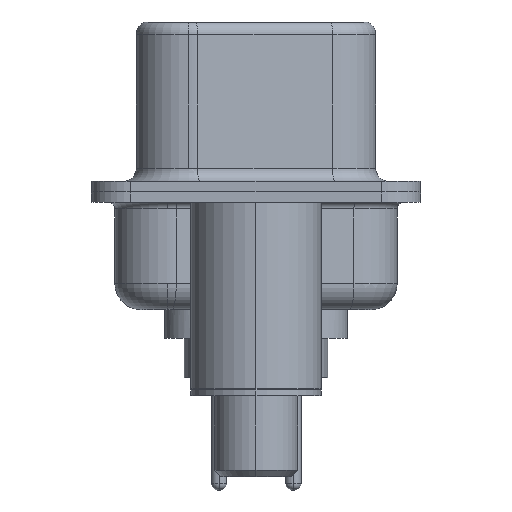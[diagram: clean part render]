
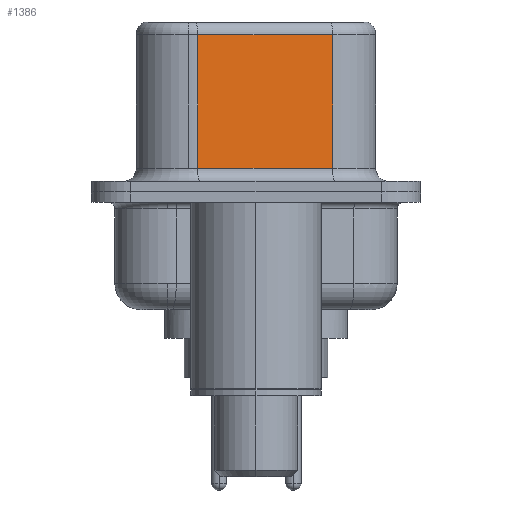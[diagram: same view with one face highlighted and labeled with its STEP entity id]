
A CAD part, left-side view. The second image highlights one B-rep face of the part: STEP entity #1386.
In plain terms, the highlighted planar face has unit normal (-0.985, -0.174, 0).
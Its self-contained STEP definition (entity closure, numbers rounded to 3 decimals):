
#341 = CARTESIAN_POINT ( 'NONE',  ( 4.565, -2.927, 0.9 ) ) ;
#1203 = LINE ( 'NONE', #9097, #8037 ) ;
#1386 = ADVANCED_FACE ( 'NONE', ( #8898 ), #8149, .F. ) ;
#2580 = CARTESIAN_POINT ( 'NONE',  ( 4.565, -2.927, 0.9 ) ) ;
#3601 = EDGE_CURVE ( 'NONE', #10204, #7075, #12284, .T. ) ;
#5334 = CARTESIAN_POINT ( 'NONE',  ( 3.655, 2.233, 0.9 ) ) ;
#5649 = VECTOR ( 'NONE', #14198, 1000. ) ;
#5680 = VERTEX_POINT ( 'NONE', #341 ) ;
#6180 = VECTOR ( 'NONE', #11380, 1000. ) ;
#6309 = EDGE_CURVE ( 'NONE', #14719, #10204, #1203, .T. ) ;
#7025 = DIRECTION ( 'NONE',  ( -0.174, 0.985, 0. ) ) ;
#7038 = DIRECTION ( 'NONE',  ( -0.174, 0.985, 0. ) ) ;
#7075 = VERTEX_POINT ( 'NONE', #5334 ) ;
#7458 = ORIENTED_EDGE ( 'NONE', *, *, #8129, .T. ) ;
#8037 = VECTOR ( 'NONE', #7038, 1000. ) ;
#8125 = EDGE_CURVE ( 'NONE', #14719, #5680, #12794, .T. ) ;
#8129 = EDGE_CURVE ( 'NONE', #7075, #5680, #9552, .T. ) ;
#8149 = PLANE ( 'NONE',  #8208 ) ;
#8208 = AXIS2_PLACEMENT_3D ( 'NONE', #15344, #13433, #7025 ) ;
#8898 = FACE_OUTER_BOUND ( 'NONE', #9405, .T. ) ;
#8985 = ORIENTED_EDGE ( 'NONE', *, *, #8125, .F. ) ;
#9097 = CARTESIAN_POINT ( 'NONE',  ( 4.565, -2.927, 6.02 ) ) ;
#9405 = EDGE_LOOP ( 'NONE', ( #8985, #15335, #15974, #7458 ) ) ;
#9552 = LINE ( 'NONE', #2580, #12402 ) ;
#10204 = VERTEX_POINT ( 'NONE', #10597 ) ;
#10597 = CARTESIAN_POINT ( 'NONE',  ( 3.655, 2.233, 6.02 ) ) ;
#11380 = DIRECTION ( 'NONE',  ( 0., 0., -1. ) ) ;
#12284 = LINE ( 'NONE', #16064, #5649 ) ;
#12402 = VECTOR ( 'NONE', #12637, 1000. ) ;
#12637 = DIRECTION ( 'NONE',  ( 0.174, -0.985, 0. ) ) ;
#12794 = LINE ( 'NONE', #16260, #6180 ) ;
#13433 = DIRECTION ( 'NONE',  ( 0.985, 0.174, 0. ) ) ;
#14048 = CARTESIAN_POINT ( 'NONE',  ( 4.565, -2.927, 6.02 ) ) ;
#14198 = DIRECTION ( 'NONE',  ( 0., 0., -1. ) ) ;
#14719 = VERTEX_POINT ( 'NONE', #14048 ) ;
#15335 = ORIENTED_EDGE ( 'NONE', *, *, #6309, .T. ) ;
#15344 = CARTESIAN_POINT ( 'NONE',  ( 4.565, -2.927, 6.52 ) ) ;
#15974 = ORIENTED_EDGE ( 'NONE', *, *, #3601, .T. ) ;
#16064 = CARTESIAN_POINT ( 'NONE',  ( 3.655, 2.233, 6.52 ) ) ;
#16260 = CARTESIAN_POINT ( 'NONE',  ( 4.565, -2.927, 6.52 ) ) ;
